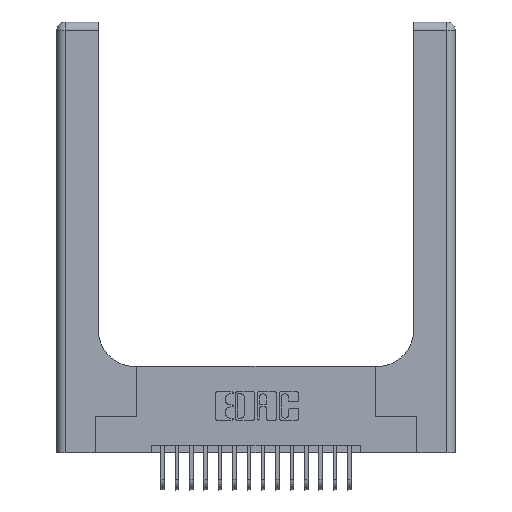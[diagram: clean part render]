
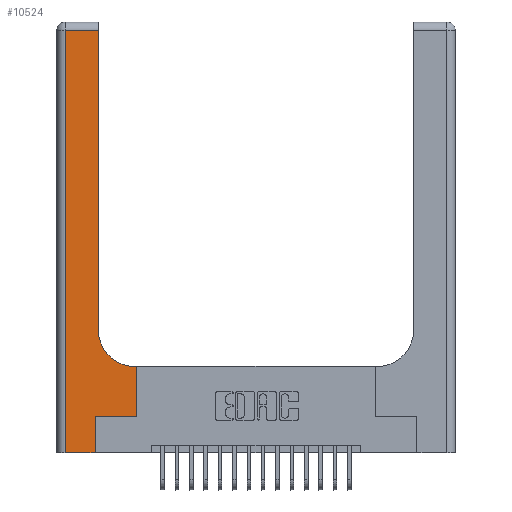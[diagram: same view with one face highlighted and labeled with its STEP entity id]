
A CAD part, top view. The second image highlights one B-rep face of the part: STEP entity #10524.
In plain terms, the highlighted planar face has unit normal (0, 0, 1).
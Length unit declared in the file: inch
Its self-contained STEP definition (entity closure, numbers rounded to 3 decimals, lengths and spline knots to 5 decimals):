
#312 = DIRECTION ( 'NONE',  ( 1., 0., 0. ) ) ;
#349 = VERTEX_POINT ( 'NONE', #6302 ) ;
#531 = DIRECTION ( 'NONE',  ( 0., 0., -1. ) ) ;
#691 = EDGE_CURVE ( 'NONE', #1280, #14637, #13171, .T. ) ;
#1280 = VERTEX_POINT ( 'NONE', #20360 ) ;
#1332 = CARTESIAN_POINT ( 'NONE',  ( 0.2915, 0.85, 0.37 ) ) ;
#1588 = VECTOR ( 'NONE', #20224, 39.37008 ) ;
#1720 = VECTOR ( 'NONE', #20563, 39.37008 ) ;
#1986 = ORIENTED_EDGE ( 'NONE', *, *, #8748, .T. ) ;
#2714 = AXIS2_PLACEMENT_3D ( 'NONE', #11309, #6522, #19699 ) ;
#3222 = CARTESIAN_POINT ( 'NONE',  ( 0.269, 0., 0.37 ) ) ;
#3280 = CARTESIAN_POINT ( 'NONE',  ( 0.5585, 0.25, 0.37 ) ) ;
#3493 = EDGE_LOOP ( 'NONE', ( #17226, #1986, #4627, #15698, #3767, #7322, #19632, #4868, #18702 ) ) ;
#3689 = CARTESIAN_POINT ( 'NONE',  ( 0.5415, 0.85, 0.37 ) ) ;
#3767 = ORIENTED_EDGE ( 'NONE', *, *, #17626, .T. ) ;
#4627 = ORIENTED_EDGE ( 'NONE', *, *, #7881, .T. ) ;
#4868 = ORIENTED_EDGE ( 'NONE', *, *, #8844, .T. ) ;
#5060 = VERTEX_POINT ( 'NONE', #20609 ) ;
#5721 = EDGE_CURVE ( 'NONE', #14084, #13358, #18748, .T. ) ;
#5898 = DIRECTION ( 'NONE',  ( 1., 0., 0. ) ) ;
#6107 = DIRECTION ( 'NONE',  ( 1., 0., 0. ) ) ;
#6108 = CARTESIAN_POINT ( 'NONE',  ( 0.06, 3., 0.37 ) ) ;
#6302 = CARTESIAN_POINT ( 'NONE',  ( 0.5415, 0.6, 0.37 ) ) ;
#6522 = DIRECTION ( 'NONE',  ( 0., 0., -1. ) ) ;
#7322 = ORIENTED_EDGE ( 'NONE', *, *, #8231, .T. ) ;
#7807 = LINE ( 'NONE', #17901, #9636 ) ;
#7881 = EDGE_CURVE ( 'NONE', #14729, #1280, #11657, .T. ) ;
#8231 = EDGE_CURVE ( 'NONE', #10578, #17161, #10892, .T. ) ;
#8449 = EDGE_CURVE ( 'NONE', #349, #14084, #9337, .T. ) ;
#8591 = AXIS2_PLACEMENT_3D ( 'NONE', #3689, #531, #312 ) ;
#8748 = EDGE_CURVE ( 'NONE', #13358, #14729, #19504, .T. ) ;
#8844 = EDGE_CURVE ( 'NONE', #5060, #349, #14489, .T. ) ;
#9178 = CARTESIAN_POINT ( 'NONE',  ( 0., 0., 0.37 ) ) ;
#9337 = CIRCLE ( 'NONE', #8591, 0.25 ) ;
#9636 = VECTOR ( 'NONE', #10984, 39.37008 ) ;
#9937 = CARTESIAN_POINT ( 'NONE',  ( 0.06, 2.94, 0.37 ) ) ;
#10079 = DIRECTION ( 'NONE',  ( 0., 1., 0. ) ) ;
#10377 = DIRECTION ( 'NONE',  ( -1., 0., 0. ) ) ;
#10524 = ADVANCED_FACE ( 'NONE', ( #13380 ), #14645, .F. ) ;
#10578 = VERTEX_POINT ( 'NONE', #10915 ) ;
#10892 = LINE ( 'NONE', #12550, #16883 ) ;
#10915 = CARTESIAN_POINT ( 'NONE',  ( 0.269, 0.25, 0.37 ) ) ;
#10917 = VECTOR ( 'NONE', #10079, 39.37008 ) ;
#10984 = DIRECTION ( 'NONE',  ( 0., 1., 0. ) ) ;
#11091 = CARTESIAN_POINT ( 'NONE',  ( 0.2915, 2.94, 0.37 ) ) ;
#11309 = CARTESIAN_POINT ( 'NONE',  ( 0., 3., 0.37 ) ) ;
#11657 = LINE ( 'NONE', #6108, #17162 ) ;
#12550 = CARTESIAN_POINT ( 'NONE',  ( 0.269, 0.25, 0.37 ) ) ;
#12719 = EDGE_CURVE ( 'NONE', #17161, #5060, #19363, .T. ) ;
#13171 = LINE ( 'NONE', #9178, #20767 ) ;
#13358 = VERTEX_POINT ( 'NONE', #11091 ) ;
#13380 = FACE_OUTER_BOUND ( 'NONE', #3493, .T. ) ;
#14084 = VERTEX_POINT ( 'NONE', #1332 ) ;
#14489 = LINE ( 'NONE', #16851, #1720 ) ;
#14637 = VERTEX_POINT ( 'NONE', #3222 ) ;
#14645 = PLANE ( 'NONE',  #2714 ) ;
#14729 = VERTEX_POINT ( 'NONE', #9937 ) ;
#15010 = CARTESIAN_POINT ( 'NONE',  ( 0.2915, 3., 0.37 ) ) ;
#15698 = ORIENTED_EDGE ( 'NONE', *, *, #691, .T. ) ;
#15821 = VECTOR ( 'NONE', #10377, 39.37008 ) ;
#16851 = CARTESIAN_POINT ( 'NONE',  ( 0.2915, 0.6, 0.37 ) ) ;
#16883 = VECTOR ( 'NONE', #6107, 39.37008 ) ;
#17161 = VERTEX_POINT ( 'NONE', #3280 ) ;
#17162 = VECTOR ( 'NONE', #20723, 39.37008 ) ;
#17226 = ORIENTED_EDGE ( 'NONE', *, *, #5721, .T. ) ;
#17626 = EDGE_CURVE ( 'NONE', #14637, #10578, #7807, .T. ) ;
#17901 = CARTESIAN_POINT ( 'NONE',  ( 0.269, 0., 0.37 ) ) ;
#18401 = CARTESIAN_POINT ( 'NONE',  ( 0.5585, 0.25, 0.37 ) ) ;
#18702 = ORIENTED_EDGE ( 'NONE', *, *, #8449, .T. ) ;
#18748 = LINE ( 'NONE', #15010, #10917 ) ;
#19363 = LINE ( 'NONE', #18401, #1588 ) ;
#19504 = LINE ( 'NONE', #20205, #15821 ) ;
#19632 = ORIENTED_EDGE ( 'NONE', *, *, #12719, .T. ) ;
#19699 = DIRECTION ( 'NONE',  ( -1., 0., 0. ) ) ;
#20205 = CARTESIAN_POINT ( 'NONE',  ( 0., 2.94, 0.37 ) ) ;
#20224 = DIRECTION ( 'NONE',  ( 0., 1., 0. ) ) ;
#20360 = CARTESIAN_POINT ( 'NONE',  ( 0.06, 0., 0.37 ) ) ;
#20563 = DIRECTION ( 'NONE',  ( -1., 0., 0. ) ) ;
#20609 = CARTESIAN_POINT ( 'NONE',  ( 0.5585, 0.6, 0.37 ) ) ;
#20723 = DIRECTION ( 'NONE',  ( 0., -1., 0. ) ) ;
#20767 = VECTOR ( 'NONE', #5898, 39.37008 ) ;
